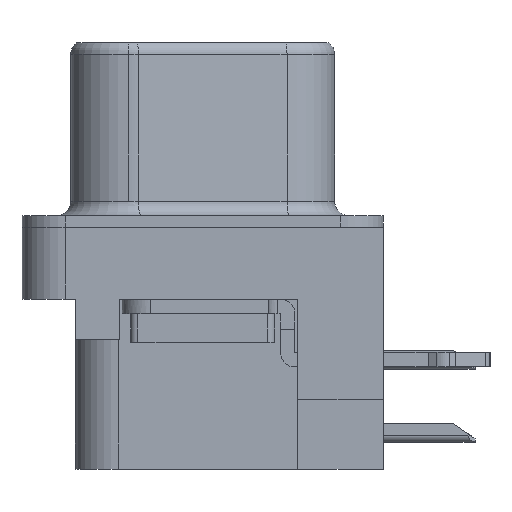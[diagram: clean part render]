
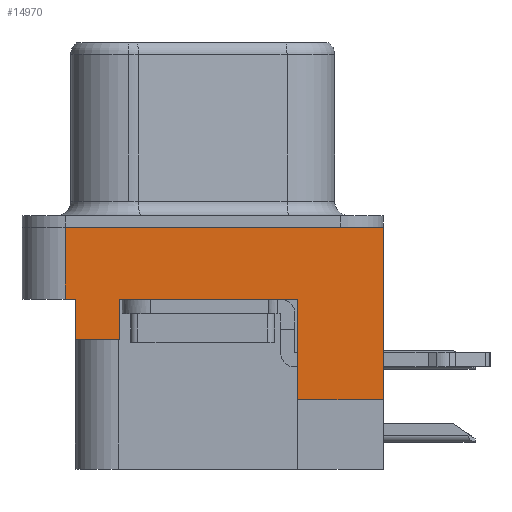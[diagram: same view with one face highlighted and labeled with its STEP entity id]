
A CAD part, left-side view. The second image highlights one B-rep face of the part: STEP entity #14970.
In plain terms, the highlighted planar face has unit normal (-1, 0, 0).
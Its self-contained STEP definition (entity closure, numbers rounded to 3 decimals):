
#183 = CARTESIAN_POINT ( 'NONE',  ( -2.935, -6.275, -6. ) ) ;
#458 = ORIENTED_EDGE ( 'NONE', *, *, #2018, .F. ) ;
#1214 = EDGE_CURVE ( 'NONE', #9713, #5440, #3870, .T. ) ;
#1297 = ORIENTED_EDGE ( 'NONE', *, *, #8843, .T. ) ;
#1378 = VECTOR ( 'NONE', #7655, 1000. ) ;
#1604 = DIRECTION ( 'NONE',  ( 0., -1., 0. ) ) ;
#1749 = DIRECTION ( 'NONE',  ( -1., 0., 0. ) ) ;
#1886 = DIRECTION ( 'NONE',  ( 0., -1., 0. ) ) ;
#2018 = EDGE_CURVE ( 'NONE', #16103, #15710, #6907, .T. ) ;
#2159 = ORIENTED_EDGE ( 'NONE', *, *, #8242, .T. ) ;
#2304 = ORIENTED_EDGE ( 'NONE', *, *, #1214, .F. ) ;
#2681 = ORIENTED_EDGE ( 'NONE', *, *, #8391, .T. ) ;
#2920 = CARTESIAN_POINT ( 'NONE',  ( -2.935, -6.275, 0. ) ) ;
#2991 = VECTOR ( 'NONE', #15658, 1000. ) ;
#3509 = DIRECTION ( 'NONE',  ( 0., 0., 1. ) ) ;
#3870 = LINE ( 'NONE', #14411, #1378 ) ;
#3932 = CARTESIAN_POINT ( 'NONE',  ( -2.935, -6.275, -2.5 ) ) ;
#4082 = CARTESIAN_POINT ( 'NONE',  ( -2.935, 4.425, -2.5 ) ) ;
#4119 = VECTOR ( 'NONE', #7741, 1000. ) ;
#4682 = DIRECTION ( 'NONE',  ( 0., 0., 1. ) ) ;
#4896 = CARTESIAN_POINT ( 'NONE',  ( -2.935, 4.775, -2.5 ) ) ;
#4956 = DIRECTION ( 'NONE',  ( 0., 1., 0. ) ) ;
#4978 = ORIENTED_EDGE ( 'NONE', *, *, #11261, .F. ) ;
#5079 = VERTEX_POINT ( 'NONE', #9264 ) ;
#5440 = VERTEX_POINT ( 'NONE', #4082 ) ;
#6104 = CARTESIAN_POINT ( 'NONE',  ( -2.935, 2.895, -2.5 ) ) ;
#6301 = VERTEX_POINT ( 'NONE', #6104 ) ;
#6459 = CARTESIAN_POINT ( 'NONE',  ( -2.935, 4.425, -3.9 ) ) ;
#6770 = LINE ( 'NONE', #11357, #9731 ) ;
#6907 = LINE ( 'NONE', #2920, #2991 ) ;
#6911 = VERTEX_POINT ( 'NONE', #4896 ) ;
#7105 = CARTESIAN_POINT ( 'NONE',  ( -2.935, -6.275, -2.5 ) ) ;
#7655 = DIRECTION ( 'NONE',  ( 0., 0., 1. ) ) ;
#7741 = DIRECTION ( 'NONE',  ( 0., 1., 0. ) ) ;
#7873 = VECTOR ( 'NONE', #11665, 1000. ) ;
#7949 = CARTESIAN_POINT ( 'NONE',  ( -2.935, 2.895, -3.9 ) ) ;
#8229 = ORIENTED_EDGE ( 'NONE', *, *, #12629, .T. ) ;
#8242 = EDGE_CURVE ( 'NONE', #10245, #15710, #14717, .T. ) ;
#8391 = EDGE_CURVE ( 'NONE', #6911, #5440, #15701, .T. ) ;
#8393 = CARTESIAN_POINT ( 'NONE',  ( -2.935, 4.425, -3.9 ) ) ;
#8843 = EDGE_CURVE ( 'NONE', #15569, #6301, #15685, .T. ) ;
#9264 = CARTESIAN_POINT ( 'NONE',  ( -2.935, -3.295, -2.5 ) ) ;
#9266 = VERTEX_POINT ( 'NONE', #12427 ) ;
#9524 = CARTESIAN_POINT ( 'NONE',  ( -2.935, -6.275, -2.5 ) ) ;
#9529 = ORIENTED_EDGE ( 'NONE', *, *, #11741, .F. ) ;
#9713 = VERTEX_POINT ( 'NONE', #8393 ) ;
#9731 = VECTOR ( 'NONE', #4956, 1000. ) ;
#9795 = EDGE_CURVE ( 'NONE', #9266, #5079, #15254, .T. ) ;
#10245 = VERTEX_POINT ( 'NONE', #183 ) ;
#10331 = CARTESIAN_POINT ( 'NONE',  ( -2.935, 4.775, 0. ) ) ;
#10553 = VECTOR ( 'NONE', #3509, 1000. ) ;
#10680 = ORIENTED_EDGE ( 'NONE', *, *, #11783, .F. ) ;
#10688 = CARTESIAN_POINT ( 'NONE',  ( -2.935, -6.275, -2.5 ) ) ;
#10819 = DIRECTION ( 'NONE',  ( 0., 0., 1. ) ) ;
#10954 = LINE ( 'NONE', #12559, #10553 ) ;
#11261 = EDGE_CURVE ( 'NONE', #15569, #9713, #12206, .T. ) ;
#11357 = CARTESIAN_POINT ( 'NONE',  ( -2.935, -6.495, -6. ) ) ;
#11573 = VECTOR ( 'NONE', #1886, 1000. ) ;
#11665 = DIRECTION ( 'NONE',  ( 0., 0., 1. ) ) ;
#11741 = EDGE_CURVE ( 'NONE', #6911, #16103, #10954, .T. ) ;
#11783 = EDGE_CURVE ( 'NONE', #10245, #9266, #6770, .T. ) ;
#11921 = ORIENTED_EDGE ( 'NONE', *, *, #9795, .F. ) ;
#12206 = LINE ( 'NONE', #6459, #4119 ) ;
#12389 = CARTESIAN_POINT ( 'NONE',  ( -2.935, -3.295, -8.4 ) ) ;
#12427 = CARTESIAN_POINT ( 'NONE',  ( -2.935, -3.295, -6. ) ) ;
#12559 = CARTESIAN_POINT ( 'NONE',  ( -2.935, 4.775, -2.5 ) ) ;
#12629 = EDGE_CURVE ( 'NONE', #6301, #5079, #14992, .T. ) ;
#12696 = VECTOR ( 'NONE', #1604, 1000. ) ;
#12785 = DIRECTION ( 'NONE',  ( 0., 0., 1. ) ) ;
#13472 = AXIS2_PLACEMENT_3D ( 'NONE', #9524, #1749, #10819 ) ;
#13542 = EDGE_LOOP ( 'NONE', ( #10680, #2159, #458, #9529, #2681, #2304, #4978, #1297, #8229, #11921 ) ) ;
#14120 = FACE_OUTER_BOUND ( 'NONE', #13542, .T. ) ;
#14275 = VECTOR ( 'NONE', #4682, 1000. ) ;
#14411 = CARTESIAN_POINT ( 'NONE',  ( -2.935, 4.425, -3.9 ) ) ;
#14717 = LINE ( 'NONE', #3932, #7873 ) ;
#14970 = ADVANCED_FACE ( 'NONE', ( #14120 ), #15962, .T. ) ;
#14992 = LINE ( 'NONE', #7105, #11573 ) ;
#15254 = LINE ( 'NONE', #12389, #14275 ) ;
#15347 = CARTESIAN_POINT ( 'NONE',  ( -2.935, 2.895, -3.9 ) ) ;
#15569 = VERTEX_POINT ( 'NONE', #7949 ) ;
#15658 = DIRECTION ( 'NONE',  ( 0., -1., 0. ) ) ;
#15685 = LINE ( 'NONE', #15347, #16091 ) ;
#15701 = LINE ( 'NONE', #10688, #12696 ) ;
#15710 = VERTEX_POINT ( 'NONE', #15925 ) ;
#15925 = CARTESIAN_POINT ( 'NONE',  ( -2.935, -6.275, 0. ) ) ;
#15962 = PLANE ( 'NONE',  #13472 ) ;
#16091 = VECTOR ( 'NONE', #12785, 1000. ) ;
#16103 = VERTEX_POINT ( 'NONE', #10331 ) ;
